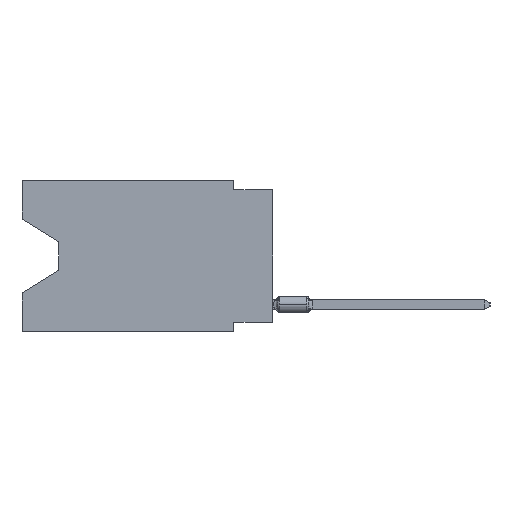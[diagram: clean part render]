
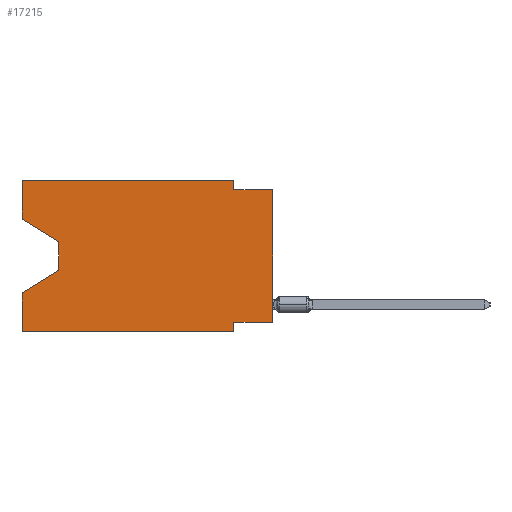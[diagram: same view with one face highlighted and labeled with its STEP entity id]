
A CAD part, left-side view. The second image highlights one B-rep face of the part: STEP entity #17215.
In plain terms, the highlighted planar face has unit normal (-1, 0, 0).
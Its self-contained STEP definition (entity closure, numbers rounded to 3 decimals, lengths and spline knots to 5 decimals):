
#33 = DIRECTION ( 'NONE',  ( 0., 0., 1. ) ) ;
#1867 = ORIENTED_EDGE ( 'NONE', *, *, #37562, .T. ) ;
#2021 = EDGE_CURVE ( 'NONE', #54489, #42430, #66312, .T. ) ;
#3441 = CARTESIAN_POINT ( 'NONE',  ( 0., 0.1, -0.39 ) ) ;
#4879 = VERTEX_POINT ( 'NONE', #22464 ) ;
#5318 = AXIS2_PLACEMENT_3D ( 'NONE', #9967, #53608, #11511 ) ;
#5638 = EDGE_CURVE ( 'NONE', #41541, #19218, #76573, .T. ) ;
#8339 = VECTOR ( 'NONE', #53675, 39.37008 ) ;
#8419 = EDGE_CURVE ( 'NONE', #18394, #8812, #37947, .T. ) ;
#8582 = CARTESIAN_POINT ( 'NONE',  ( 0., 0.1, -0.025 ) ) ;
#8812 = VERTEX_POINT ( 'NONE', #13235 ) ;
#9301 = ORIENTED_EDGE ( 'NONE', *, *, #19668, .T. ) ;
#9967 = CARTESIAN_POINT ( 'NONE',  ( 0., 0.645, 0. ) ) ;
#11511 = DIRECTION ( 'NONE',  ( 0., 0., -1. ) ) ;
#13235 = CARTESIAN_POINT ( 'NONE',  ( 0., 0.1, -0.365 ) ) ;
#13777 = DIRECTION ( 'NONE',  ( 0., 0., -1. ) ) ;
#15403 = CARTESIAN_POINT ( 'NONE',  ( 0., 0.645, -0.39 ) ) ;
#16093 = CARTESIAN_POINT ( 'NONE',  ( 0., 0.645, -0.39 ) ) ;
#16408 = DIRECTION ( 'NONE',  ( 0., -1., 0. ) ) ;
#16496 = EDGE_CURVE ( 'NONE', #42892, #42430, #49116, .T. ) ;
#16685 = EDGE_CURVE ( 'NONE', #8812, #69544, #56254, .T. ) ;
#17156 = VECTOR ( 'NONE', #30199, 39.37008 ) ;
#17215 = ADVANCED_FACE ( 'NONE', ( #34967 ), #47254, .F. ) ;
#18394 = VERTEX_POINT ( 'NONE', #22315 ) ;
#18721 = VECTOR ( 'NONE', #55015, 39.37008 ) ;
#19218 = VERTEX_POINT ( 'NONE', #67229 ) ;
#19668 = EDGE_CURVE ( 'NONE', #21634, #54489, #54823, .T. ) ;
#19744 = CARTESIAN_POINT ( 'NONE',  ( 0., 0.1, -0.39 ) ) ;
#21634 = VERTEX_POINT ( 'NONE', #33214 ) ;
#22315 = CARTESIAN_POINT ( 'NONE',  ( 0., 0., -0.365 ) ) ;
#22464 = CARTESIAN_POINT ( 'NONE',  ( 0., 0.645, -0.10025 ) ) ;
#23296 = EDGE_CURVE ( 'NONE', #75259, #38931, #40240, .T. ) ;
#23572 = ORIENTED_EDGE ( 'NONE', *, *, #16496, .F. ) ;
#23924 = CARTESIAN_POINT ( 'NONE',  ( 0., 0.645, 0. ) ) ;
#24642 = EDGE_CURVE ( 'NONE', #38931, #41541, #72772, .T. ) ;
#25077 = DIRECTION ( 'NONE',  ( 0., 0., -1. ) ) ;
#25085 = LINE ( 'NONE', #25468, #30748 ) ;
#25468 = CARTESIAN_POINT ( 'NONE',  ( 0., 0., 0. ) ) ;
#26041 = VECTOR ( 'NONE', #40014, 39.37008 ) ;
#29470 = CARTESIAN_POINT ( 'NONE',  ( 0., 0.645, -0.10025 ) ) ;
#29874 = DIRECTION ( 'NONE',  ( 0., 0., 1. ) ) ;
#30199 = DIRECTION ( 'NONE',  ( 0., 0.855, -0.519 ) ) ;
#30624 = CARTESIAN_POINT ( 'NONE',  ( 0., 0.55, -0.158 ) ) ;
#30748 = VECTOR ( 'NONE', #33, 39.37008 ) ;
#31564 = ORIENTED_EDGE ( 'NONE', *, *, #8419, .F. ) ;
#31986 = VECTOR ( 'NONE', #13777, 39.37008 ) ;
#33073 = ORIENTED_EDGE ( 'NONE', *, *, #23296, .F. ) ;
#33214 = CARTESIAN_POINT ( 'NONE',  ( 0., 0.55, -0.158 ) ) ;
#33927 = VECTOR ( 'NONE', #58665, 39.37008 ) ;
#34967 = FACE_OUTER_BOUND ( 'NONE', #69478, .T. ) ;
#35031 = LINE ( 'NONE', #29470, #8339 ) ;
#35641 = DIRECTION ( 'NONE',  ( 0., 0., 1. ) ) ;
#36314 = VECTOR ( 'NONE', #29874, 39.37008 ) ;
#36616 = CARTESIAN_POINT ( 'NONE',  ( 0., 0.1, 0. ) ) ;
#37562 = EDGE_CURVE ( 'NONE', #4879, #21634, #35031, .T. ) ;
#37781 = ORIENTED_EDGE ( 'NONE', *, *, #63526, .T. ) ;
#37947 = LINE ( 'NONE', #67320, #18721 ) ;
#38011 = ORIENTED_EDGE ( 'NONE', *, *, #51847, .F. ) ;
#38931 = VERTEX_POINT ( 'NONE', #36616 ) ;
#40014 = DIRECTION ( 'NONE',  ( 0., -1., 0. ) ) ;
#40240 = LINE ( 'NONE', #46954, #45914 ) ;
#41541 = VERTEX_POINT ( 'NONE', #8582 ) ;
#42430 = VERTEX_POINT ( 'NONE', #47531 ) ;
#42559 = LINE ( 'NONE', #23924, #36314 ) ;
#42892 = VERTEX_POINT ( 'NONE', #16093 ) ;
#43767 = CARTESIAN_POINT ( 'NONE',  ( 0., 0.1, 0. ) ) ;
#45211 = ORIENTED_EDGE ( 'NONE', *, *, #24642, .F. ) ;
#45569 = LINE ( 'NONE', #15403, #26041 ) ;
#45914 = VECTOR ( 'NONE', #16408, 39.37008 ) ;
#46954 = CARTESIAN_POINT ( 'NONE',  ( 0., 0.645, 0. ) ) ;
#47254 = PLANE ( 'NONE',  #5318 ) ;
#47531 = CARTESIAN_POINT ( 'NONE',  ( 0., 0.645, -0.28975 ) ) ;
#49116 = LINE ( 'NONE', #72551, #53443 ) ;
#51847 = EDGE_CURVE ( 'NONE', #4879, #75259, #42559, .T. ) ;
#53443 = VECTOR ( 'NONE', #35641, 39.37008 ) ;
#53608 = DIRECTION ( 'NONE',  ( 1., 0., 0. ) ) ;
#53675 = DIRECTION ( 'NONE',  ( 0., -0.855, -0.519 ) ) ;
#54217 = ORIENTED_EDGE ( 'NONE', *, *, #2021, .T. ) ;
#54489 = VERTEX_POINT ( 'NONE', #58244 ) ;
#54823 = LINE ( 'NONE', #30624, #63772 ) ;
#55015 = DIRECTION ( 'NONE',  ( 0., 1., 0. ) ) ;
#56254 = LINE ( 'NONE', #19744, #31986 ) ;
#57436 = VECTOR ( 'NONE', #77678, 39.37008 ) ;
#58244 = CARTESIAN_POINT ( 'NONE',  ( 0., 0.55, -0.232 ) ) ;
#58452 = ORIENTED_EDGE ( 'NONE', *, *, #58871, .T. ) ;
#58665 = DIRECTION ( 'NONE',  ( 0., -1., 0. ) ) ;
#58871 = EDGE_CURVE ( 'NONE', #18394, #19218, #25085, .T. ) ;
#63526 = EDGE_CURVE ( 'NONE', #42892, #69544, #45569, .T. ) ;
#63772 = VECTOR ( 'NONE', #25077, 39.37008 ) ;
#66188 = CARTESIAN_POINT ( 'NONE',  ( 0., 0., -0.025 ) ) ;
#66312 = LINE ( 'NONE', #72665, #17156 ) ;
#66732 = ORIENTED_EDGE ( 'NONE', *, *, #16685, .F. ) ;
#67229 = CARTESIAN_POINT ( 'NONE',  ( 0., 0., -0.025 ) ) ;
#67320 = CARTESIAN_POINT ( 'NONE',  ( 0., 0., -0.365 ) ) ;
#69478 = EDGE_LOOP ( 'NONE', ( #1867, #9301, #54217, #23572, #37781, #66732, #31564, #58452, #69934, #45211, #33073, #38011 ) ) ;
#69544 = VERTEX_POINT ( 'NONE', #3441 ) ;
#69934 = ORIENTED_EDGE ( 'NONE', *, *, #5638, .F. ) ;
#72551 = CARTESIAN_POINT ( 'NONE',  ( 0., 0.645, 0. ) ) ;
#72665 = CARTESIAN_POINT ( 'NONE',  ( 0., 0.55, -0.232 ) ) ;
#72772 = LINE ( 'NONE', #43767, #57436 ) ;
#74862 = CARTESIAN_POINT ( 'NONE',  ( 0., 0.645, 0. ) ) ;
#75259 = VERTEX_POINT ( 'NONE', #74862 ) ;
#76573 = LINE ( 'NONE', #66188, #33927 ) ;
#77678 = DIRECTION ( 'NONE',  ( 0., 0., -1. ) ) ;
